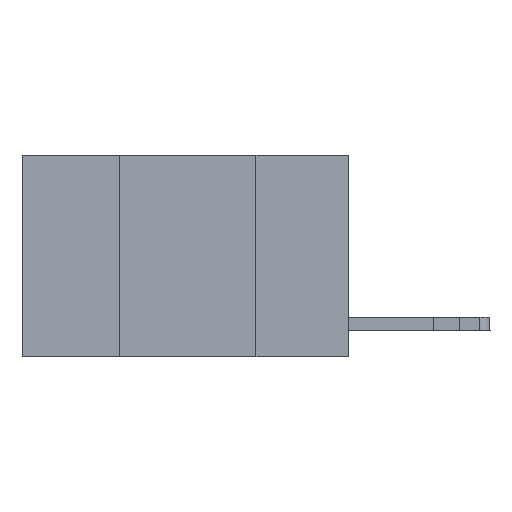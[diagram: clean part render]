
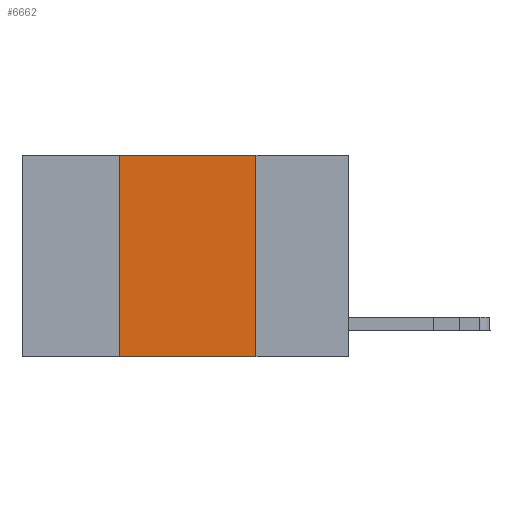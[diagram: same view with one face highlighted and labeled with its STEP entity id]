
A CAD part, left-side view. The second image highlights one B-rep face of the part: STEP entity #6662.
In plain terms, the highlighted planar face has unit normal (-1, 0, 0).
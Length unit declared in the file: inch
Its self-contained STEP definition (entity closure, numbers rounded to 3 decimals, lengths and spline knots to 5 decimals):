
#684 = VERTEX_POINT ( 'NONE', #4564 ) ;
#699 = CARTESIAN_POINT ( 'NONE',  ( 0., 0.6, 0. ) ) ;
#1046 = VERTEX_POINT ( 'NONE', #11363 ) ;
#1467 = ORIENTED_EDGE ( 'NONE', *, *, #3228, .F. ) ;
#1471 = EDGE_CURVE ( 'NONE', #10679, #684, #12642, .T. ) ;
#1803 = DIRECTION ( 'NONE',  ( 0., 0., -1. ) ) ;
#1841 = EDGE_CURVE ( 'NONE', #1046, #684, #7088, .T. ) ;
#1919 = DIRECTION ( 'NONE',  ( 0., -1., 0. ) ) ;
#2528 = CARTESIAN_POINT ( 'NONE',  ( 0., 0.42, -0.37 ) ) ;
#3008 = AXIS2_PLACEMENT_3D ( 'NONE', #699, #11174, #7201 ) ;
#3055 = PLANE ( 'NONE',  #3008 ) ;
#3228 = EDGE_CURVE ( 'NONE', #15040, #1046, #10063, .T. ) ;
#4463 = EDGE_CURVE ( 'NONE', #10679, #15040, #16417, .T. ) ;
#4564 = CARTESIAN_POINT ( 'NONE',  ( 0., 0.17, -0.37 ) ) ;
#5149 = ORIENTED_EDGE ( 'NONE', *, *, #1841, .F. ) ;
#5656 = FACE_OUTER_BOUND ( 'NONE', #7795, .T. ) ;
#6124 = CARTESIAN_POINT ( 'NONE',  ( 0., 0.42, 0. ) ) ;
#6662 = ADVANCED_FACE ( 'NONE', ( #5656 ), #3055, .F. ) ;
#7088 = LINE ( 'NONE', #7981, #13142 ) ;
#7201 = DIRECTION ( 'NONE',  ( 0., 0., -1. ) ) ;
#7795 = EDGE_LOOP ( 'NONE', ( #5149, #1467, #16490, #10461 ) ) ;
#7981 = CARTESIAN_POINT ( 'NONE',  ( 0., 0.17, 0. ) ) ;
#8995 = CARTESIAN_POINT ( 'NONE',  ( 0., 0.42, 0. ) ) ;
#9675 = VECTOR ( 'NONE', #1919, 39.37008 ) ;
#9825 = DIRECTION ( 'NONE',  ( 0., 0., 1. ) ) ;
#10063 = LINE ( 'NONE', #15514, #13740 ) ;
#10461 = ORIENTED_EDGE ( 'NONE', *, *, #1471, .T. ) ;
#10679 = VERTEX_POINT ( 'NONE', #2528 ) ;
#11174 = DIRECTION ( 'NONE',  ( 1., 0., 0. ) ) ;
#11363 = CARTESIAN_POINT ( 'NONE',  ( 0., 0.17, 0. ) ) ;
#12642 = LINE ( 'NONE', #13693, #9675 ) ;
#13142 = VECTOR ( 'NONE', #1803, 39.37008 ) ;
#13693 = CARTESIAN_POINT ( 'NONE',  ( 0., 0.6, -0.37 ) ) ;
#13740 = VECTOR ( 'NONE', #15339, 39.37008 ) ;
#14559 = VECTOR ( 'NONE', #9825, 39.37008 ) ;
#15040 = VERTEX_POINT ( 'NONE', #8995 ) ;
#15339 = DIRECTION ( 'NONE',  ( 0., -1., 0. ) ) ;
#15514 = CARTESIAN_POINT ( 'NONE',  ( 0., 0.6, 0. ) ) ;
#16417 = LINE ( 'NONE', #6124, #14559 ) ;
#16490 = ORIENTED_EDGE ( 'NONE', *, *, #4463, .F. ) ;
